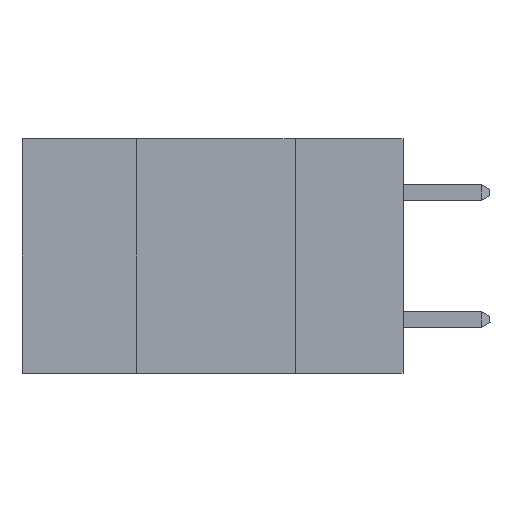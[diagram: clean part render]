
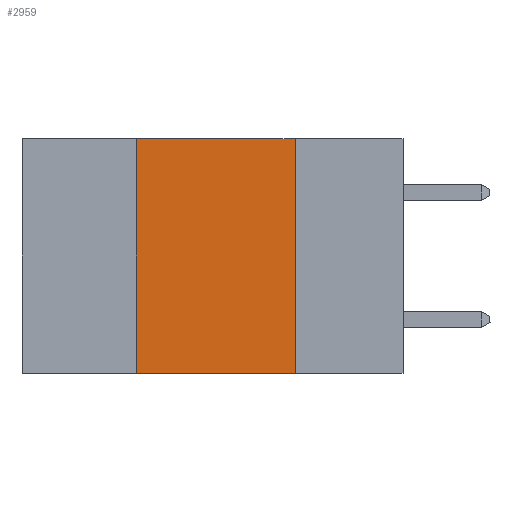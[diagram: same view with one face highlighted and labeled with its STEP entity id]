
A CAD part, left-side view. The second image highlights one B-rep face of the part: STEP entity #2959.
In plain terms, the highlighted planar face has unit normal (-1, 0, 0).
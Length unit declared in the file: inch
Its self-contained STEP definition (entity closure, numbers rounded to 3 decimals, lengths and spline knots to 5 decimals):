
#569 = VERTEX_POINT ( 'NONE', #2616 ) ;
#954 = CARTESIAN_POINT ( 'NONE',  ( 0., 0.42, 0. ) ) ;
#2494 = ORIENTED_EDGE ( 'NONE', *, *, #14041, .F. ) ;
#2560 = LINE ( 'NONE', #954, #6696 ) ;
#2616 = CARTESIAN_POINT ( 'NONE',  ( 0., 0.17, 0. ) ) ;
#2922 = DIRECTION ( 'NONE',  ( 0., -1., 0. ) ) ;
#2959 = ADVANCED_FACE ( 'NONE', ( #7193 ), #11753, .F. ) ;
#3182 = VECTOR ( 'NONE', #2922, 39.37008 ) ;
#3306 = VERTEX_POINT ( 'NONE', #11707 ) ;
#5419 = EDGE_CURVE ( 'NONE', #3306, #18209, #8519, .T. ) ;
#5662 = DIRECTION ( 'NONE',  ( 0., 0., 1. ) ) ;
#6156 = AXIS2_PLACEMENT_3D ( 'NONE', #11851, #17894, #13260 ) ;
#6696 = VECTOR ( 'NONE', #5662, 39.37008 ) ;
#7193 = FACE_OUTER_BOUND ( 'NONE', #11541, .T. ) ;
#7208 = CARTESIAN_POINT ( 'NONE',  ( 0., 0.17, -0.37 ) ) ;
#7599 = VECTOR ( 'NONE', #13295, 39.37008 ) ;
#8519 = LINE ( 'NONE', #12888, #13005 ) ;
#8648 = LINE ( 'NONE', #9983, #7599 ) ;
#9032 = CARTESIAN_POINT ( 'NONE',  ( 0., 0.6, 0. ) ) ;
#9371 = VERTEX_POINT ( 'NONE', #11426 ) ;
#9983 = CARTESIAN_POINT ( 'NONE',  ( 0., 0.17, 0. ) ) ;
#11140 = EDGE_CURVE ( 'NONE', #569, #18209, #8648, .T. ) ;
#11426 = CARTESIAN_POINT ( 'NONE',  ( 0., 0.42, 0. ) ) ;
#11541 = EDGE_LOOP ( 'NONE', ( #13728, #2494, #12282, #13048 ) ) ;
#11707 = CARTESIAN_POINT ( 'NONE',  ( 0., 0.42, -0.37 ) ) ;
#11753 = PLANE ( 'NONE',  #6156 ) ;
#11851 = CARTESIAN_POINT ( 'NONE',  ( 0., 0.6, 0. ) ) ;
#12051 = EDGE_CURVE ( 'NONE', #3306, #9371, #2560, .T. ) ;
#12282 = ORIENTED_EDGE ( 'NONE', *, *, #12051, .F. ) ;
#12888 = CARTESIAN_POINT ( 'NONE',  ( 0., 0.6, -0.37 ) ) ;
#13005 = VECTOR ( 'NONE', #13079, 39.37008 ) ;
#13048 = ORIENTED_EDGE ( 'NONE', *, *, #5419, .T. ) ;
#13079 = DIRECTION ( 'NONE',  ( 0., -1., 0. ) ) ;
#13260 = DIRECTION ( 'NONE',  ( 0., 0., -1. ) ) ;
#13295 = DIRECTION ( 'NONE',  ( 0., 0., -1. ) ) ;
#13728 = ORIENTED_EDGE ( 'NONE', *, *, #11140, .F. ) ;
#14041 = EDGE_CURVE ( 'NONE', #9371, #569, #19836, .T. ) ;
#17894 = DIRECTION ( 'NONE',  ( 1., 0., 0. ) ) ;
#18209 = VERTEX_POINT ( 'NONE', #7208 ) ;
#19836 = LINE ( 'NONE', #9032, #3182 ) ;
